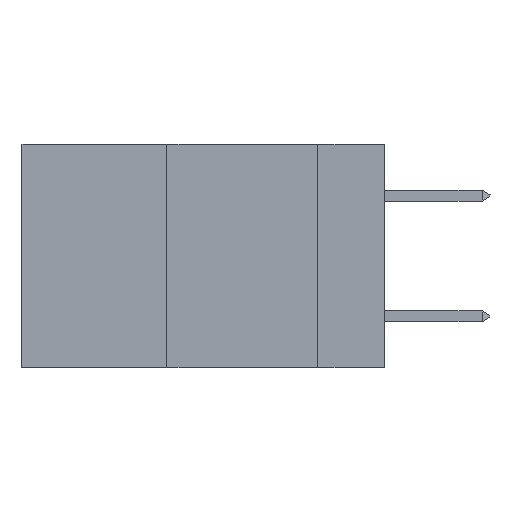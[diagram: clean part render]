
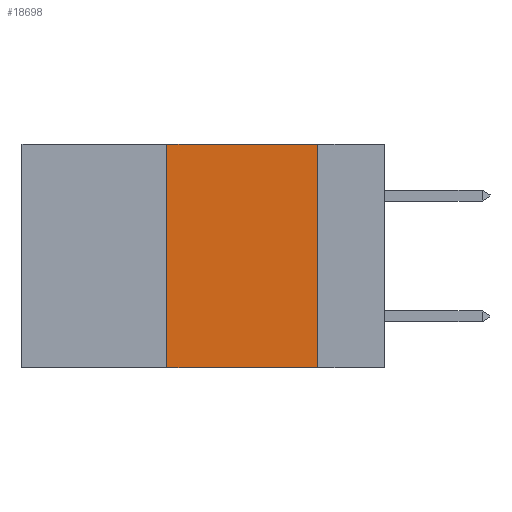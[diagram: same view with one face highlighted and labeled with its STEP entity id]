
A CAD part, left-side view. The second image highlights one B-rep face of the part: STEP entity #18698.
In plain terms, the highlighted planar face has unit normal (-1, 0, 0).
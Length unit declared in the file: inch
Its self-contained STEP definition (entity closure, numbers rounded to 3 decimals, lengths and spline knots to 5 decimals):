
#1046 = LINE ( 'NONE', #2462, #25942 ) ;
#1453 = PLANE ( 'NONE',  #9654 ) ;
#1953 = VERTEX_POINT ( 'NONE', #11382 ) ;
#1967 = DIRECTION ( 'NONE',  ( 0., -1., 0. ) ) ;
#2462 = CARTESIAN_POINT ( 'NONE',  ( 0., 0.6, -0.37 ) ) ;
#3626 = CARTESIAN_POINT ( 'NONE',  ( 0., 0.36, 0. ) ) ;
#5622 = DIRECTION ( 'NONE',  ( 0., 0., 1. ) ) ;
#5677 = DIRECTION ( 'NONE',  ( 1., 0., 0. ) ) ;
#5727 = VECTOR ( 'NONE', #5622, 39.37008 ) ;
#6084 = CARTESIAN_POINT ( 'NONE',  ( 0., 0.36, -0.37 ) ) ;
#6134 = EDGE_CURVE ( 'NONE', #19523, #13200, #1046, .T. ) ;
#6990 = DIRECTION ( 'NONE',  ( 0., 0., -1. ) ) ;
#7223 = EDGE_CURVE ( 'NONE', #19523, #15254, #11058, .T. ) ;
#7402 = ORIENTED_EDGE ( 'NONE', *, *, #23096, .F. ) ;
#9654 = AXIS2_PLACEMENT_3D ( 'NONE', #21694, #5677, #23887 ) ;
#9904 = EDGE_CURVE ( 'NONE', #1953, #13200, #21622, .T. ) ;
#10065 = ORIENTED_EDGE ( 'NONE', *, *, #6134, .T. ) ;
#11058 = LINE ( 'NONE', #3626, #5727 ) ;
#11382 = CARTESIAN_POINT ( 'NONE',  ( 0., 0.11, 0. ) ) ;
#12158 = FACE_OUTER_BOUND ( 'NONE', #22136, .T. ) ;
#12925 = ORIENTED_EDGE ( 'NONE', *, *, #7223, .F. ) ;
#13200 = VERTEX_POINT ( 'NONE', #13893 ) ;
#13893 = CARTESIAN_POINT ( 'NONE',  ( 0., 0.11, -0.37 ) ) ;
#15254 = VERTEX_POINT ( 'NONE', #18614 ) ;
#16246 = VECTOR ( 'NONE', #6990, 39.37008 ) ;
#16693 = ORIENTED_EDGE ( 'NONE', *, *, #9904, .F. ) ;
#18614 = CARTESIAN_POINT ( 'NONE',  ( 0., 0.36, 0. ) ) ;
#18698 = ADVANCED_FACE ( 'NONE', ( #12158 ), #1453, .F. ) ;
#19523 = VERTEX_POINT ( 'NONE', #6084 ) ;
#21369 = CARTESIAN_POINT ( 'NONE',  ( 0., 0.11, 0. ) ) ;
#21622 = LINE ( 'NONE', #21369, #16246 ) ;
#21694 = CARTESIAN_POINT ( 'NONE',  ( 0., 0.6, 0. ) ) ;
#22136 = EDGE_LOOP ( 'NONE', ( #16693, #7402, #12925, #10065 ) ) ;
#22679 = VECTOR ( 'NONE', #1967, 39.37008 ) ;
#23096 = EDGE_CURVE ( 'NONE', #15254, #1953, #24572, .T. ) ;
#23887 = DIRECTION ( 'NONE',  ( 0., 0., -1. ) ) ;
#24208 = CARTESIAN_POINT ( 'NONE',  ( 0., 0.6, 0. ) ) ;
#24447 = DIRECTION ( 'NONE',  ( 0., -1., 0. ) ) ;
#24572 = LINE ( 'NONE', #24208, #22679 ) ;
#25942 = VECTOR ( 'NONE', #24447, 39.37008 ) ;
